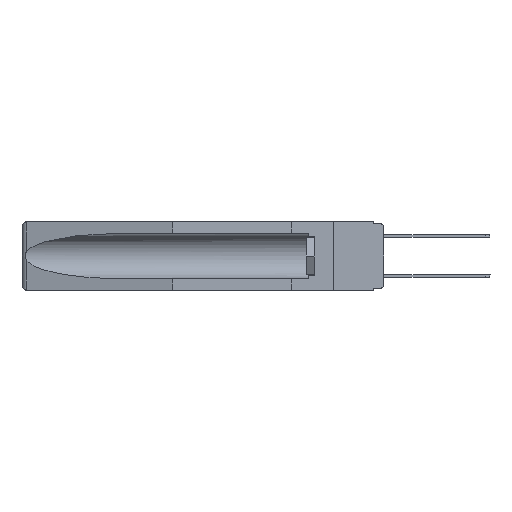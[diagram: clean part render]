
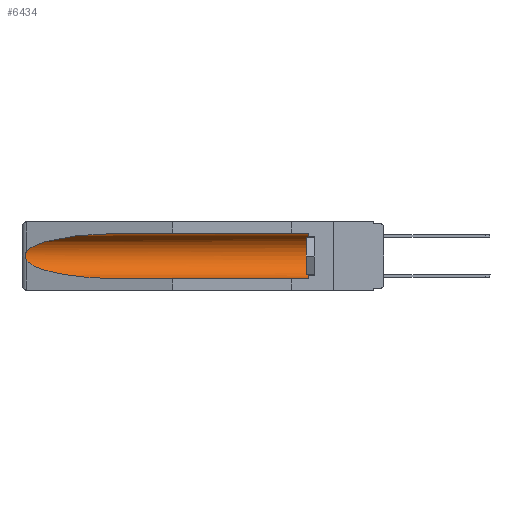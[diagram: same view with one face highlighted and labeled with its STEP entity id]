
A CAD part, left-side view. The second image highlights one B-rep face of the part: STEP entity #6434.
In plain terms, the highlighted cylindrical face has radius 2.857 mm (diameter 5.715 mm), a partial arc.
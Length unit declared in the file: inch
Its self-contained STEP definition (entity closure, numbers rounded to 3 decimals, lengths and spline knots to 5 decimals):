
#294 = FACE_OUTER_BOUND ( 'NONE', #13659, .T. ) ;
#295 = CARTESIAN_POINT ( 'NONE',  ( 0.26537, 1.52718, -0.14972 ) ) ;
#727 = CARTESIAN_POINT ( 'NONE',  ( 0.155, 1.07973, -0.284 ) ) ;
#1108 = CARTESIAN_POINT ( 'NONE',  ( 0.155, 0.126, -0.1715 ) ) ;
#1318 = CARTESIAN_POINT ( 'NONE',  ( 0.2675, 1.53308, -0.16763 ) ) ;
#1407 = CARTESIAN_POINT ( 'NONE',  ( 0.26537, 1.52718, -0.14972 ) ) ;
#1509 = CARTESIAN_POINT ( 'NONE',  ( 0.26537, 1.52718, -0.14972 ) ) ;
#1535 = CARTESIAN_POINT ( 'NONE',  ( 0.26537, 1.52718, -0.19328 ) ) ;
#1598 = DIRECTION ( 'NONE',  ( 0., 1., 0. ) ) ;
#1749 = DIRECTION ( 'NONE',  ( 0., 0., 1. ) ) ;
#2082 = ORIENTED_EDGE ( 'NONE', *, *, #16198, .F. ) ;
#2770 = CARTESIAN_POINT ( 'NONE',  ( 0.155, 0.126, -0.284 ) ) ;
#2871 = CARTESIAN_POINT ( 'NONE',  ( 0.26537, 1.52718, -0.19328 ) ) ;
#3628 = ORIENTED_EDGE ( 'NONE', *, *, #4049, .T. ) ;
#4049 = EDGE_CURVE ( 'NONE', #8806, #10511, #11921, .T. ) ;
#4341 = CARTESIAN_POINT ( 'NONE',  ( 0.26655, 1.53094, -0.18657 ) ) ;
#4879 = AXIS2_PLACEMENT_3D ( 'NONE', #14689, #12074, #1749 ) ;
#4968 = CIRCLE ( 'NONE', #17279, 0.1125 ) ;
#5270 = DIRECTION ( 'NONE',  ( 0., 1., 0. ) ) ;
#5606 = VERTEX_POINT ( 'NONE', #12578 ) ;
#5790 = CARTESIAN_POINT ( 'NONE',  ( 0.2675, 1.53308, -0.17534 ) ) ;
#5962 = CARTESIAN_POINT ( 'NONE',  ( 0.155, 1.07973, -0.059 ) ) ;
#6260 = CARTESIAN_POINT ( 'NONE',  ( 0.21114, 1.30732, -0.059 ) ) ;
#6434 = ADVANCED_FACE ( 'NONE', ( #294 ), #16428, .F. ) ;
#6546 = ORIENTED_EDGE ( 'NONE', *, *, #14389, .T. ) ;
#6651 = CARTESIAN_POINT ( 'NONE',  ( 0.21114, 1.30732, -0.284 ) ) ;
#6898 =( BOUNDED_CURVE ( )  B_SPLINE_CURVE ( 3, ( #10960, #16866, #6651, #727 ),
 .UNSPECIFIED., .F., .T. ) 
 B_SPLINE_CURVE_WITH_KNOTS ( ( 4, 4 ),
 ( 0.1948, 1.5708 ),
 .UNSPECIFIED. ) 
 CURVE ( )  GEOMETRIC_REPRESENTATION_ITEM ( )  RATIONAL_B_SPLINE_CURVE ( ( 1., 0.848, 0.848, 1. ) ) 
 REPRESENTATION_ITEM ( '' )  );
#7079 = EDGE_CURVE ( 'NONE', #10511, #9264, #12786, .T. ) ;
#7418 = DIRECTION ( 'NONE',  ( 0., 0., 1. ) ) ;
#7793 = CARTESIAN_POINT ( 'NONE',  ( 0.155, 1.07973, -0.059 ) ) ;
#8344 = ORIENTED_EDGE ( 'NONE', *, *, #18806, .T. ) ;
#8385 = VERTEX_POINT ( 'NONE', #1535 ) ;
#8415 = VECTOR ( 'NONE', #5270, 39.37008 ) ;
#8477 = CARTESIAN_POINT ( 'NONE',  ( 0.26654, 1.53092, -0.15636 ) ) ;
#8806 = VERTEX_POINT ( 'NONE', #8838 ) ;
#8838 = CARTESIAN_POINT ( 'NONE',  ( 0.155, 0.126, -0.059 ) ) ;
#9264 = VERTEX_POINT ( 'NONE', #295 ) ;
#9775 = LINE ( 'NONE', #18489, #8415 ) ;
#10107 = CARTESIAN_POINT ( 'NONE',  ( 0.26597, 1.52961, -0.15275 ) ) ;
#10381 = CARTESIAN_POINT ( 'NONE',  ( 0.2673, 1.53269, -0.17917 ) ) ;
#10511 = VERTEX_POINT ( 'NONE', #5962 ) ;
#10522 = VERTEX_POINT ( 'NONE', #2770 ) ;
#10960 = CARTESIAN_POINT ( 'NONE',  ( 0.26537, 1.52718, -0.19328 ) ) ;
#10969 = ORIENTED_EDGE ( 'NONE', *, *, #18916, .T. ) ;
#11921 = LINE ( 'NONE', #19098, #15015 ) ;
#11922 = CARTESIAN_POINT ( 'NONE',  ( 0.25451, 1.48313, -0.09465 ) ) ;
#12074 = DIRECTION ( 'NONE',  ( 0., 1., 0. ) ) ;
#12578 = CARTESIAN_POINT ( 'NONE',  ( 0.155, 1.07973, -0.284 ) ) ;
#12786 =( BOUNDED_CURVE ( )  B_SPLINE_CURVE ( 3, ( #7793, #6260, #11922, #1509 ),
 .UNSPECIFIED., .F., .T. ) 
 B_SPLINE_CURVE_WITH_KNOTS ( ( 4, 4 ),
 ( 4.71239, 6.08839 ),
 .UNSPECIFIED. ) 
 CURVE ( )  GEOMETRIC_REPRESENTATION_ITEM ( )  RATIONAL_B_SPLINE_CURVE ( ( 1., 0.848, 0.848, 1. ) ) 
 REPRESENTATION_ITEM ( '' )  );
#13659 = EDGE_LOOP ( 'NONE', ( #15383, #10969, #8344, #2082, #6546, #3628 ) ) ;
#14389 = EDGE_CURVE ( 'NONE', #10522, #8806, #4968, .T. ) ;
#14428 = B_SPLINE_CURVE_WITH_KNOTS ( 'NONE', 3,
 ( #1407, #10107, #8477, #16089, #1318, #5790, #10381, #4341, #18807, #2871 ),
 .UNSPECIFIED., .F., .F.,
 ( 4, 2, 2, 2, 4 ),
 ( 0., 0.00029, 0.00058, 0.00087, 0.00117 ),
 .UNSPECIFIED. ) ;
#14689 = CARTESIAN_POINT ( 'NONE',  ( 0.155, -0.30754, -0.1715 ) ) ;
#15015 = VECTOR ( 'NONE', #1598, 39.37008 ) ;
#15383 = ORIENTED_EDGE ( 'NONE', *, *, #7079, .T. ) ;
#16089 = CARTESIAN_POINT ( 'NONE',  ( 0.2673, 1.5327, -0.16383 ) ) ;
#16171 = DIRECTION ( 'NONE',  ( 0., -1., 0. ) ) ;
#16198 = EDGE_CURVE ( 'NONE', #10522, #5606, #9775, .T. ) ;
#16428 = CYLINDRICAL_SURFACE ( 'NONE', #4879, 0.1125 ) ;
#16866 = CARTESIAN_POINT ( 'NONE',  ( 0.25451, 1.48313, -0.24835 ) ) ;
#17279 = AXIS2_PLACEMENT_3D ( 'NONE', #1108, #16171, #7418 ) ;
#18489 = CARTESIAN_POINT ( 'NONE',  ( 0.155, -0.30754, -0.284 ) ) ;
#18806 = EDGE_CURVE ( 'NONE', #8385, #5606, #6898, .T. ) ;
#18807 = CARTESIAN_POINT ( 'NONE',  ( 0.26597, 1.5296, -0.19026 ) ) ;
#18916 = EDGE_CURVE ( 'NONE', #9264, #8385, #14428, .T. ) ;
#19098 = CARTESIAN_POINT ( 'NONE',  ( 0.155, -0.30754, -0.059 ) ) ;
